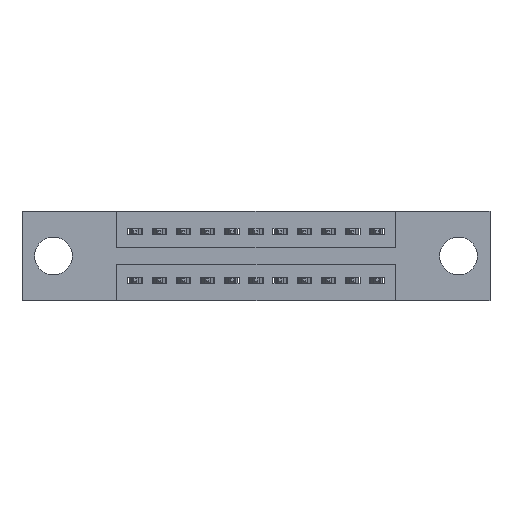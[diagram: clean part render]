
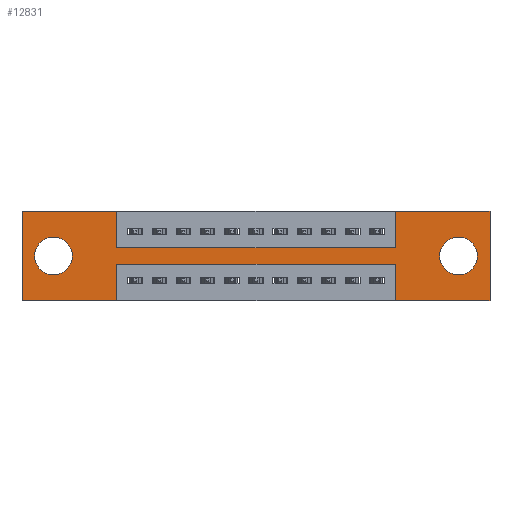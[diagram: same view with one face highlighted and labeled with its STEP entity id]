
A CAD part, front view. The second image highlights one B-rep face of the part: STEP entity #12831.
In plain terms, the highlighted planar face has unit normal (0, -1, 0).
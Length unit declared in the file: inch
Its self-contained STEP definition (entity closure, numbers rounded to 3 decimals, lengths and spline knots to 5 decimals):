
#10 = VECTOR ( 'NONE', #1344, 39.37008 ) ;
#12 = CARTESIAN_POINT ( 'NONE',  ( 0.3925, 0., -0.37 ) ) ;
#56 = EDGE_CURVE ( 'NONE', #1793, #6775, #2690, .T. ) ;
#96 = VECTOR ( 'NONE', #2912, 39.37008 ) ;
#110 = EDGE_CURVE ( 'NONE', #3951, #3119, #6645, .T. ) ;
#475 = DIRECTION ( 'NONE',  ( 0., 1., 0. ) ) ;
#575 = CARTESIAN_POINT ( 'NONE',  ( 1.935, 0., 0. ) ) ;
#737 = LINE ( 'NONE', #7786, #5607 ) ;
#762 = ORIENTED_EDGE ( 'NONE', *, *, #110, .F. ) ;
#981 = LINE ( 'NONE', #10857, #8660 ) ;
#1061 = ORIENTED_EDGE ( 'NONE', *, *, #2046, .F. ) ;
#1167 = DIRECTION ( 'NONE',  ( 0., 0., -1. ) ) ;
#1285 = CARTESIAN_POINT ( 'NONE',  ( 0.3925, 0., -0.22 ) ) ;
#1344 = DIRECTION ( 'NONE',  ( 1., 0., 0. ) ) ;
#1373 = LINE ( 'NONE', #11655, #7798 ) ;
#1510 = EDGE_LOOP ( 'NONE', ( #5246, #11532 ) ) ;
#1547 = AXIS2_PLACEMENT_3D ( 'NONE', #7312, #475, #2345 ) ;
#1563 = CARTESIAN_POINT ( 'NONE',  ( 0., 0., 0. ) ) ;
#1622 = EDGE_CURVE ( 'NONE', #10110, #12269, #6451, .T. ) ;
#1691 = DIRECTION ( 'NONE',  ( 0., 0., 1. ) ) ;
#1767 = CIRCLE ( 'NONE', #1974, 0.078 ) ;
#1793 = VERTEX_POINT ( 'NONE', #3759 ) ;
#1799 = CARTESIAN_POINT ( 'NONE',  ( 0.13, 0., -0.185 ) ) ;
#1974 = AXIS2_PLACEMENT_3D ( 'NONE', #2421, #12478, #9663 ) ;
#2008 = EDGE_CURVE ( 'NONE', #5476, #9023, #10141, .T. ) ;
#2046 = EDGE_CURVE ( 'NONE', #5814, #12334, #6368, .T. ) ;
#2117 = CARTESIAN_POINT ( 'NONE',  ( 0., 0., 0. ) ) ;
#2153 = CARTESIAN_POINT ( 'NONE',  ( 0., 0., 0. ) ) ;
#2168 = VECTOR ( 'NONE', #1691, 39.37008 ) ;
#2187 = DIRECTION ( 'NONE',  ( 0., 0., 1. ) ) ;
#2305 = FACE_BOUND ( 'NONE', #1510, .T. ) ;
#2345 = DIRECTION ( 'NONE',  ( 0., 0., -1. ) ) ;
#2360 = VECTOR ( 'NONE', #13232, 39.37008 ) ;
#2369 = DIRECTION ( 'NONE',  ( 0., -1., 0. ) ) ;
#2421 = CARTESIAN_POINT ( 'NONE',  ( 1.805, 0., -0.185 ) ) ;
#2568 = VERTEX_POINT ( 'NONE', #4192 ) ;
#2616 = DIRECTION ( 'NONE',  ( 0., 0., -1. ) ) ;
#2690 = LINE ( 'NONE', #1563, #2168 ) ;
#2773 = LINE ( 'NONE', #12996, #10978 ) ;
#2912 = DIRECTION ( 'NONE',  ( 0., 0., -1. ) ) ;
#2977 = CARTESIAN_POINT ( 'NONE',  ( 1.5425, 0., -0.15 ) ) ;
#3066 = CARTESIAN_POINT ( 'NONE',  ( 0.13, 0., -0.263 ) ) ;
#3110 = CARTESIAN_POINT ( 'NONE',  ( 0.3925, 0., -0.15 ) ) ;
#3119 = VERTEX_POINT ( 'NONE', #7827 ) ;
#3237 = DIRECTION ( 'NONE',  ( 0., 1., 0. ) ) ;
#3299 = EDGE_CURVE ( 'NONE', #11409, #1793, #2773, .T. ) ;
#3537 = CARTESIAN_POINT ( 'NONE',  ( 0.13, 0., -0.107 ) ) ;
#3614 = CARTESIAN_POINT ( 'NONE',  ( 0., 0., -0.37 ) ) ;
#3638 = VERTEX_POINT ( 'NONE', #11016 ) ;
#3707 = CIRCLE ( 'NONE', #12718, 0.078 ) ;
#3759 = CARTESIAN_POINT ( 'NONE',  ( 0., 0., -0.37 ) ) ;
#3947 = EDGE_LOOP ( 'NONE', ( #6475, #7935 ) ) ;
#3951 = VERTEX_POINT ( 'NONE', #10391 ) ;
#4127 = VERTEX_POINT ( 'NONE', #3537 ) ;
#4192 = CARTESIAN_POINT ( 'NONE',  ( 1.805, 0., -0.263 ) ) ;
#4298 = CIRCLE ( 'NONE', #1547, 0.078 ) ;
#4849 = EDGE_CURVE ( 'NONE', #6775, #3638, #10482, .T. ) ;
#4855 = EDGE_CURVE ( 'NONE', #4127, #11833, #3707, .T. ) ;
#5064 = CARTESIAN_POINT ( 'NONE',  ( 1.935, 0., 0. ) ) ;
#5246 = ORIENTED_EDGE ( 'NONE', *, *, #10404, .T. ) ;
#5329 = VERTEX_POINT ( 'NONE', #8535 ) ;
#5388 = FACE_BOUND ( 'NONE', #3947, .T. ) ;
#5457 = DIRECTION ( 'NONE',  ( -1., 0., 0. ) ) ;
#5476 = VERTEX_POINT ( 'NONE', #11197 ) ;
#5571 = EDGE_CURVE ( 'NONE', #12334, #5476, #981, .T. ) ;
#5607 = VECTOR ( 'NONE', #2616, 39.37008 ) ;
#5625 = ORIENTED_EDGE ( 'NONE', *, *, #12469, .F. ) ;
#5642 = VECTOR ( 'NONE', #7492, 39.37008 ) ;
#5804 = VECTOR ( 'NONE', #7666, 39.37008 ) ;
#5814 = VERTEX_POINT ( 'NONE', #3110 ) ;
#5831 = EDGE_CURVE ( 'NONE', #9023, #3951, #10362, .T. ) ;
#5886 = DIRECTION ( 'NONE',  ( 0., 1., 0. ) ) ;
#6368 = LINE ( 'NONE', #8530, #10 ) ;
#6451 = LINE ( 'NONE', #1285, #8340 ) ;
#6471 = EDGE_LOOP ( 'NONE', ( #12519, #7265, #5625, #762, #7655, #8586, #8829, #1061, #6786, #8271, #12237, #9683 ) ) ;
#6475 = ORIENTED_EDGE ( 'NONE', *, *, #4855, .T. ) ;
#6645 = LINE ( 'NONE', #3614, #5804 ) ;
#6775 = VERTEX_POINT ( 'NONE', #2153 ) ;
#6786 = ORIENTED_EDGE ( 'NONE', *, *, #11932, .F. ) ;
#7105 = CARTESIAN_POINT ( 'NONE',  ( 0., 0., 0. ) ) ;
#7265 = ORIENTED_EDGE ( 'NONE', *, *, #1622, .F. ) ;
#7312 = CARTESIAN_POINT ( 'NONE',  ( 1.805, 0., -0.185 ) ) ;
#7335 = DIRECTION ( 'NONE',  ( 0., 0., 1. ) ) ;
#7492 = DIRECTION ( 'NONE',  ( 0., 0., -1. ) ) ;
#7655 = ORIENTED_EDGE ( 'NONE', *, *, #5831, .F. ) ;
#7666 = DIRECTION ( 'NONE',  ( -1., 0., 0. ) ) ;
#7786 = CARTESIAN_POINT ( 'NONE',  ( 0.3925, 0., -0.37 ) ) ;
#7798 = VECTOR ( 'NONE', #2187, 39.37008 ) ;
#7827 = CARTESIAN_POINT ( 'NONE',  ( 1.5425, 0., -0.37 ) ) ;
#7935 = ORIENTED_EDGE ( 'NONE', *, *, #8827, .T. ) ;
#8271 = ORIENTED_EDGE ( 'NONE', *, *, #4849, .F. ) ;
#8340 = VECTOR ( 'NONE', #5457, 39.37008 ) ;
#8347 = PLANE ( 'NONE',  #10156 ) ;
#8482 = DIRECTION ( 'NONE',  ( 1., 0., 0. ) ) ;
#8530 = CARTESIAN_POINT ( 'NONE',  ( 0.3925, 0., -0.15 ) ) ;
#8535 = CARTESIAN_POINT ( 'NONE',  ( 1.805, 0., -0.107 ) ) ;
#8586 = ORIENTED_EDGE ( 'NONE', *, *, #2008, .F. ) ;
#8660 = VECTOR ( 'NONE', #12251, 39.37008 ) ;
#8827 = EDGE_CURVE ( 'NONE', #11833, #4127, #13086, .T. ) ;
#8829 = ORIENTED_EDGE ( 'NONE', *, *, #5571, .F. ) ;
#9023 = VERTEX_POINT ( 'NONE', #575 ) ;
#9237 = CARTESIAN_POINT ( 'NONE',  ( 0.3925, 0., -0.22 ) ) ;
#9359 = FACE_OUTER_BOUND ( 'NONE', #6471, .T. ) ;
#9386 = LINE ( 'NONE', #11528, #5642 ) ;
#9663 = DIRECTION ( 'NONE',  ( 0., 0., -1. ) ) ;
#9683 = ORIENTED_EDGE ( 'NONE', *, *, #3299, .F. ) ;
#10102 = DIRECTION ( 'NONE',  ( 0., 0., 1. ) ) ;
#10110 = VERTEX_POINT ( 'NONE', #11899 ) ;
#10141 = LINE ( 'NONE', #7105, #2360 ) ;
#10156 = AXIS2_PLACEMENT_3D ( 'NONE', #12635, #2369, #1167 ) ;
#10349 = EDGE_CURVE ( 'NONE', #2568, #5329, #1767, .T. ) ;
#10362 = LINE ( 'NONE', #5064, #96 ) ;
#10391 = CARTESIAN_POINT ( 'NONE',  ( 1.935, 0., -0.37 ) ) ;
#10404 = EDGE_CURVE ( 'NONE', #5329, #2568, #4298, .T. ) ;
#10482 = LINE ( 'NONE', #2117, #11870 ) ;
#10523 = EDGE_CURVE ( 'NONE', #12269, #11409, #737, .T. ) ;
#10857 = CARTESIAN_POINT ( 'NONE',  ( 1.5425, 0., 0. ) ) ;
#10978 = VECTOR ( 'NONE', #13247, 39.37008 ) ;
#11016 = CARTESIAN_POINT ( 'NONE',  ( 0.3925, 0., 0. ) ) ;
#11197 = CARTESIAN_POINT ( 'NONE',  ( 1.5425, 0., 0. ) ) ;
#11409 = VERTEX_POINT ( 'NONE', #12 ) ;
#11441 = CARTESIAN_POINT ( 'NONE',  ( 0.13, 0., -0.185 ) ) ;
#11528 = CARTESIAN_POINT ( 'NONE',  ( 0.3925, 0., 0. ) ) ;
#11532 = ORIENTED_EDGE ( 'NONE', *, *, #10349, .T. ) ;
#11655 = CARTESIAN_POINT ( 'NONE',  ( 1.5425, 0., -0.37 ) ) ;
#11807 = AXIS2_PLACEMENT_3D ( 'NONE', #1799, #5886, #10102 ) ;
#11833 = VERTEX_POINT ( 'NONE', #3066 ) ;
#11870 = VECTOR ( 'NONE', #8482, 39.37008 ) ;
#11899 = CARTESIAN_POINT ( 'NONE',  ( 1.5425, 0., -0.22 ) ) ;
#11932 = EDGE_CURVE ( 'NONE', #3638, #5814, #9386, .T. ) ;
#12237 = ORIENTED_EDGE ( 'NONE', *, *, #56, .F. ) ;
#12251 = DIRECTION ( 'NONE',  ( 0., 0., 1. ) ) ;
#12269 = VERTEX_POINT ( 'NONE', #9237 ) ;
#12334 = VERTEX_POINT ( 'NONE', #2977 ) ;
#12469 = EDGE_CURVE ( 'NONE', #3119, #10110, #1373, .T. ) ;
#12478 = DIRECTION ( 'NONE',  ( 0., 1., 0. ) ) ;
#12519 = ORIENTED_EDGE ( 'NONE', *, *, #10523, .F. ) ;
#12635 = CARTESIAN_POINT ( 'NONE',  ( 0., 0., -0.37 ) ) ;
#12718 = AXIS2_PLACEMENT_3D ( 'NONE', #11441, #3237, #7335 ) ;
#12831 = ADVANCED_FACE ( 'NONE', ( #2305, #5388, #9359 ), #8347, .T. ) ;
#12996 = CARTESIAN_POINT ( 'NONE',  ( 0., 0., -0.37 ) ) ;
#13086 = CIRCLE ( 'NONE', #11807, 0.078 ) ;
#13232 = DIRECTION ( 'NONE',  ( 1., 0., 0. ) ) ;
#13247 = DIRECTION ( 'NONE',  ( -1., 0., 0. ) ) ;
